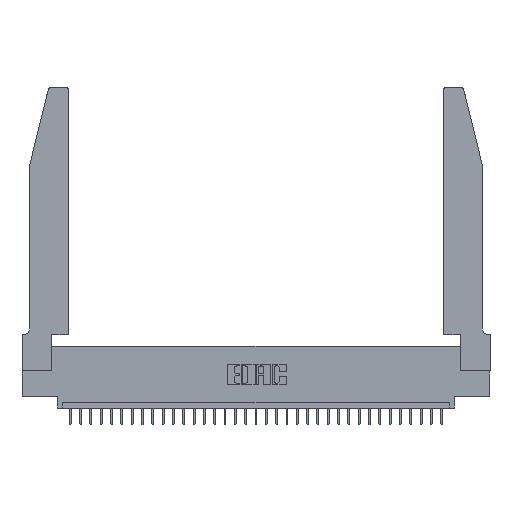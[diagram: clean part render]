
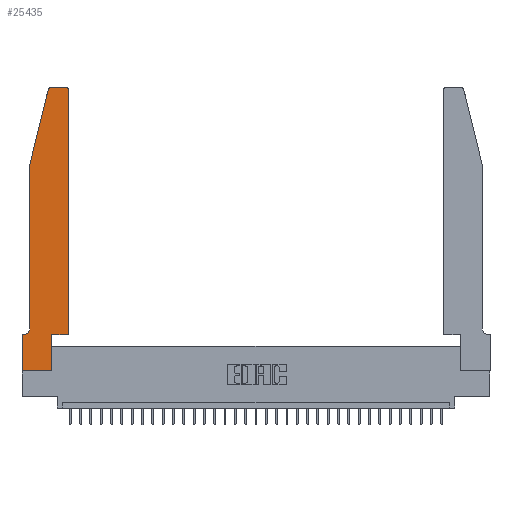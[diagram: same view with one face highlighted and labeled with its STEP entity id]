
A CAD part, top view. The second image highlights one B-rep face of the part: STEP entity #25435.
In plain terms, the highlighted planar face has unit normal (0, 0, 1).
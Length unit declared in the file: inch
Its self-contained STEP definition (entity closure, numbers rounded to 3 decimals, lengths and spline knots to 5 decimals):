
#112 = ORIENTED_EDGE ( 'NONE', *, *, #25796, .T. ) ;
#220 = VERTEX_POINT ( 'NONE', #14911 ) ;
#676 = DIRECTION ( 'NONE',  ( 0., -1., 0. ) ) ;
#788 = CARTESIAN_POINT ( 'NONE',  ( 0.0755, 2., 0.37 ) ) ;
#1217 = ORIENTED_EDGE ( 'NONE', *, *, #11038, .T. ) ;
#1532 = CARTESIAN_POINT ( 'NONE',  ( 0.2865, 0.35, 0.37 ) ) ;
#1588 = ORIENTED_EDGE ( 'NONE', *, *, #14468, .T. ) ;
#1622 = CARTESIAN_POINT ( 'NONE',  ( 0.284, 2.75, 0.37 ) ) ;
#2374 = LINE ( 'NONE', #32037, #25008 ) ;
#2429 = EDGE_CURVE ( 'NONE', #18181, #14200, #24820, .T. ) ;
#2881 = CARTESIAN_POINT ( 'NONE',  ( 0.0755, 0.35, 0.37 ) ) ;
#3124 = VERTEX_POINT ( 'NONE', #26202 ) ;
#3134 = CARTESIAN_POINT ( 'NONE',  ( 0.4505, 0.35, 0.37 ) ) ;
#3228 = LINE ( 'NONE', #7595, #14890 ) ;
#3821 = VERTEX_POINT ( 'NONE', #1622 ) ;
#4510 = VERTEX_POINT ( 'NONE', #14780 ) ;
#4684 = PLANE ( 'NONE',  #22189 ) ;
#4842 = LINE ( 'NONE', #17220, #26672 ) ;
#5046 = DIRECTION ( 'NONE',  ( -1., 0., 0. ) ) ;
#5130 = DIRECTION ( 'NONE',  ( -1., 0., 0. ) ) ;
#5272 = VECTOR ( 'NONE', #676, 39.37008 ) ;
#5300 = CARTESIAN_POINT ( 'NONE',  ( 0.25487, 2.72718, 0.37 ) ) ;
#5483 = EDGE_CURVE ( 'NONE', #30233, #4510, #4842, .T. ) ;
#5738 = EDGE_CURVE ( 'NONE', #22198, #3821, #3228, .T. ) ;
#5834 = CARTESIAN_POINT ( 'NONE',  ( 0.284, 2.72, 0.37 ) ) ;
#5949 = DIRECTION ( 'NONE',  ( 1., 0., 0. ) ) ;
#6527 = DIRECTION ( 'NONE',  ( 1., 0., 0. ) ) ;
#6628 = EDGE_CURVE ( 'NONE', #3821, #18181, #10830, .T. ) ;
#7521 = VECTOR ( 'NONE', #33107, 39.37008 ) ;
#7595 = CARTESIAN_POINT ( 'NONE',  ( 0.2605, 2.75, 0.37 ) ) ;
#8531 = VERTEX_POINT ( 'NONE', #1532 ) ;
#8536 = LINE ( 'NONE', #16071, #15353 ) ;
#9297 = LINE ( 'NONE', #21094, #19369 ) ;
#9418 = ORIENTED_EDGE ( 'NONE', *, *, #25378, .T. ) ;
#9745 = VERTEX_POINT ( 'NONE', #23331 ) ;
#9767 = EDGE_CURVE ( 'NONE', #30432, #31890, #8536, .T. ) ;
#10103 = DIRECTION ( 'NONE',  ( 1., 0., 0. ) ) ;
#10579 = CARTESIAN_POINT ( 'NONE',  ( 0.4205, 2.72, 0.37 ) ) ;
#10830 = CIRCLE ( 'NONE', #16386, 0.03 ) ;
#10840 = DIRECTION ( 'NONE',  ( 1., 0., 0. ) ) ;
#11038 = EDGE_CURVE ( 'NONE', #4510, #9745, #2374, .T. ) ;
#12790 = ORIENTED_EDGE ( 'NONE', *, *, #32620, .T. ) ;
#13667 = ORIENTED_EDGE ( 'NONE', *, *, #5738, .T. ) ;
#14200 = VERTEX_POINT ( 'NONE', #20199 ) ;
#14468 = EDGE_CURVE ( 'NONE', #14200, #3124, #27114, .T. ) ;
#14780 = CARTESIAN_POINT ( 'NONE',  ( 0., 0., 0.37 ) ) ;
#14890 = VECTOR ( 'NONE', #5130, 39.37008 ) ;
#14911 = CARTESIAN_POINT ( 'NONE',  ( 0.0055, 0.35, 0.37 ) ) ;
#15353 = VECTOR ( 'NONE', #18544, 39.37008 ) ;
#16071 = CARTESIAN_POINT ( 'NONE',  ( 0.4505, 0.35, 0.37 ) ) ;
#16386 = AXIS2_PLACEMENT_3D ( 'NONE', #5834, #16625, #5949 ) ;
#16625 = DIRECTION ( 'NONE',  ( 0., 0., 1. ) ) ;
#16732 = LINE ( 'NONE', #2881, #20364 ) ;
#17220 = CARTESIAN_POINT ( 'NONE',  ( 0., 0., 0.37 ) ) ;
#17241 = CIRCLE ( 'NONE', #30214, 0.07 ) ;
#17416 = DIRECTION ( 'NONE',  ( 0., 0., -1. ) ) ;
#17918 = VECTOR ( 'NONE', #28881, 39.37008 ) ;
#18181 = VERTEX_POINT ( 'NONE', #5300 ) ;
#18544 = DIRECTION ( 'NONE',  ( 0., 1., 0. ) ) ;
#19369 = VECTOR ( 'NONE', #10840, 39.37008 ) ;
#20023 = DIRECTION ( 'NONE',  ( -1., 0., 0. ) ) ;
#20199 = CARTESIAN_POINT ( 'NONE',  ( 0.0755, 2., 0.37 ) ) ;
#20220 = CARTESIAN_POINT ( 'NONE',  ( 0., 0.35, 0.37 ) ) ;
#20364 = VECTOR ( 'NONE', #5046, 39.37008 ) ;
#20451 = CARTESIAN_POINT ( 'NONE',  ( 0.2865, 0.35, 0.37 ) ) ;
#21094 = CARTESIAN_POINT ( 'NONE',  ( 0.4505, 0.35, 0.37 ) ) ;
#21269 = LINE ( 'NONE', #20451, #7521 ) ;
#21479 = ORIENTED_EDGE ( 'NONE', *, *, #27397, .T. ) ;
#22189 = AXIS2_PLACEMENT_3D ( 'NONE', #20220, #22852, #10103 ) ;
#22198 = VERTEX_POINT ( 'NONE', #25883 ) ;
#22852 = DIRECTION ( 'NONE',  ( 0., 0., 1. ) ) ;
#23118 = CARTESIAN_POINT ( 'NONE',  ( 0., 0.35, 0.37 ) ) ;
#23331 = CARTESIAN_POINT ( 'NONE',  ( 0.2865, 0., 0.37 ) ) ;
#23396 = CARTESIAN_POINT ( 'NONE',  ( 0.4505, 2.72, 0.37 ) ) ;
#23710 = ORIENTED_EDGE ( 'NONE', *, *, #33113, .T. ) ;
#24820 = LINE ( 'NONE', #32514, #17918 ) ;
#25008 = VECTOR ( 'NONE', #6527, 39.37008 ) ;
#25202 = ORIENTED_EDGE ( 'NONE', *, *, #5483, .T. ) ;
#25378 = EDGE_CURVE ( 'NONE', #9745, #8531, #21269, .T. ) ;
#25435 = ADVANCED_FACE ( 'NONE', ( #30937 ), #4684, .T. ) ;
#25796 = EDGE_CURVE ( 'NONE', #220, #30233, #16732, .T. ) ;
#25883 = CARTESIAN_POINT ( 'NONE',  ( 0.4205, 2.75, 0.37 ) ) ;
#26153 = DIRECTION ( 'NONE',  ( 1., 0., 0. ) ) ;
#26202 = CARTESIAN_POINT ( 'NONE',  ( 0.0755, 0.42, 0.37 ) ) ;
#26240 = AXIS2_PLACEMENT_3D ( 'NONE', #10579, #28968, #26153 ) ;
#26672 = VECTOR ( 'NONE', #30788, 39.37008 ) ;
#27114 = LINE ( 'NONE', #788, #5272 ) ;
#27376 = ORIENTED_EDGE ( 'NONE', *, *, #9767, .T. ) ;
#27397 = EDGE_CURVE ( 'NONE', #3124, #220, #17241, .T. ) ;
#28229 = CIRCLE ( 'NONE', #26240, 0.03 ) ;
#28881 = DIRECTION ( 'NONE',  ( -0.239, -0.971, 0. ) ) ;
#28968 = DIRECTION ( 'NONE',  ( 0., 0., 1. ) ) ;
#29473 = ORIENTED_EDGE ( 'NONE', *, *, #2429, .T. ) ;
#30214 = AXIS2_PLACEMENT_3D ( 'NONE', #32907, #17416, #20023 ) ;
#30233 = VERTEX_POINT ( 'NONE', #23118 ) ;
#30432 = VERTEX_POINT ( 'NONE', #3134 ) ;
#30600 = ORIENTED_EDGE ( 'NONE', *, *, #6628, .T. ) ;
#30788 = DIRECTION ( 'NONE',  ( 0., -1., 0. ) ) ;
#30937 = FACE_OUTER_BOUND ( 'NONE', #32350, .T. ) ;
#31890 = VERTEX_POINT ( 'NONE', #23396 ) ;
#32037 = CARTESIAN_POINT ( 'NONE',  ( 0., 0., 0.37 ) ) ;
#32350 = EDGE_LOOP ( 'NONE', ( #13667, #30600, #29473, #1588, #21479, #112, #25202, #1217, #9418, #12790, #27376, #23710 ) ) ;
#32514 = CARTESIAN_POINT ( 'NONE',  ( 0.0755, 2., 0.37 ) ) ;
#32620 = EDGE_CURVE ( 'NONE', #8531, #30432, #9297, .T. ) ;
#32907 = CARTESIAN_POINT ( 'NONE',  ( 0.0055, 0.42, 0.37 ) ) ;
#33107 = DIRECTION ( 'NONE',  ( 0., 1., 0. ) ) ;
#33113 = EDGE_CURVE ( 'NONE', #31890, #22198, #28229, .T. ) ;
